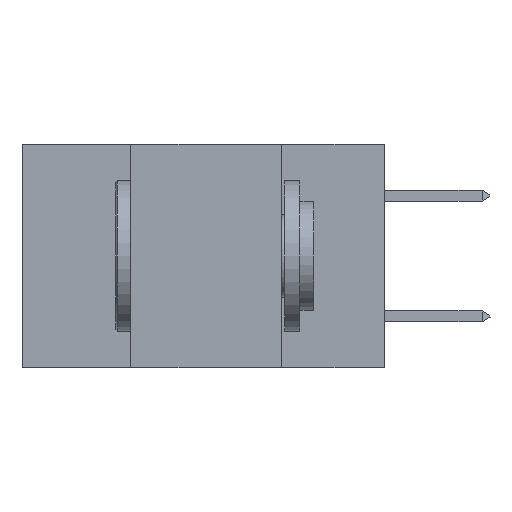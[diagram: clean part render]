
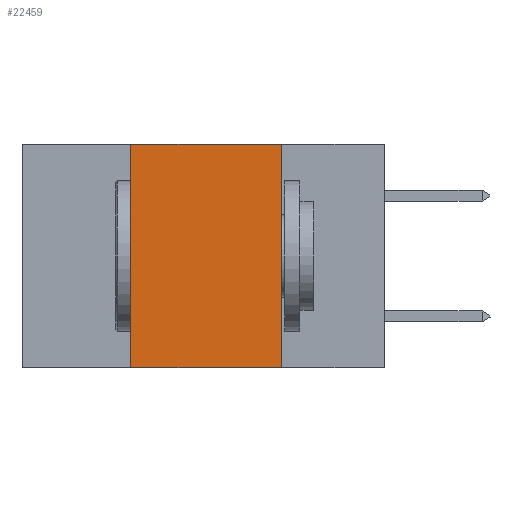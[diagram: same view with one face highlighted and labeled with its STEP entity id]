
A CAD part, left-side view. The second image highlights one B-rep face of the part: STEP entity #22459.
In plain terms, the highlighted planar face has unit normal (-1, 0, 0).
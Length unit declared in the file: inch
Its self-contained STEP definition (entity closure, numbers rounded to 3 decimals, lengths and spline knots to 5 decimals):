
#873 = LINE ( 'NONE', #25288, #9762 ) ;
#1353 = EDGE_CURVE ( 'NONE', #3779, #5149, #873, .T. ) ;
#2006 = CARTESIAN_POINT ( 'NONE',  ( 0., 0.6, 0. ) ) ;
#2845 = VERTEX_POINT ( 'NONE', #12413 ) ;
#3779 = VERTEX_POINT ( 'NONE', #20628 ) ;
#4001 = EDGE_CURVE ( 'NONE', #22722, #3779, #24430, .T. ) ;
#5149 = VERTEX_POINT ( 'NONE', #20703 ) ;
#5752 = VECTOR ( 'NONE', #41455, 39.37008 ) ;
#6653 = DIRECTION ( 'NONE',  ( 0., 0., 1. ) ) ;
#9762 = VECTOR ( 'NONE', #21986, 39.37008 ) ;
#11736 = CARTESIAN_POINT ( 'NONE',  ( 0., 0.42, 0. ) ) ;
#12413 = CARTESIAN_POINT ( 'NONE',  ( 0., 0.42, -0.37 ) ) ;
#13778 = VECTOR ( 'NONE', #6653, 39.37008 ) ;
#14039 = PLANE ( 'NONE',  #39167 ) ;
#15725 = ORIENTED_EDGE ( 'NONE', *, *, #20161, .T. ) ;
#15850 = LINE ( 'NONE', #26395, #13778 ) ;
#18760 = ORIENTED_EDGE ( 'NONE', *, *, #4001, .F. ) ;
#20161 = EDGE_CURVE ( 'NONE', #2845, #5149, #31944, .T. ) ;
#20608 = DIRECTION ( 'NONE',  ( 0., 0., -1. ) ) ;
#20628 = CARTESIAN_POINT ( 'NONE',  ( 0., 0.17, 0. ) ) ;
#20703 = CARTESIAN_POINT ( 'NONE',  ( 0., 0.17, -0.37 ) ) ;
#21986 = DIRECTION ( 'NONE',  ( 0., 0., -1. ) ) ;
#22459 = ADVANCED_FACE ( 'NONE', ( #36259 ), #14039, .F. ) ;
#22722 = VERTEX_POINT ( 'NONE', #11736 ) ;
#23468 = EDGE_CURVE ( 'NONE', #2845, #22722, #15850, .T. ) ;
#23849 = ORIENTED_EDGE ( 'NONE', *, *, #1353, .F. ) ;
#24430 = LINE ( 'NONE', #2006, #41568 ) ;
#25088 = DIRECTION ( 'NONE',  ( 0., -1., 0. ) ) ;
#25288 = CARTESIAN_POINT ( 'NONE',  ( 0., 0.17, 0. ) ) ;
#26395 = CARTESIAN_POINT ( 'NONE',  ( 0., 0.42, 0. ) ) ;
#30049 = ORIENTED_EDGE ( 'NONE', *, *, #23468, .F. ) ;
#31944 = LINE ( 'NONE', #38211, #5752 ) ;
#36259 = FACE_OUTER_BOUND ( 'NONE', #40569, .T. ) ;
#36783 = CARTESIAN_POINT ( 'NONE',  ( 0., 0.6, 0. ) ) ;
#38211 = CARTESIAN_POINT ( 'NONE',  ( 0., 0.6, -0.37 ) ) ;
#39167 = AXIS2_PLACEMENT_3D ( 'NONE', #36783, #40004, #20608 ) ;
#40004 = DIRECTION ( 'NONE',  ( 1., 0., 0. ) ) ;
#40569 = EDGE_LOOP ( 'NONE', ( #23849, #18760, #30049, #15725 ) ) ;
#41455 = DIRECTION ( 'NONE',  ( 0., -1., 0. ) ) ;
#41568 = VECTOR ( 'NONE', #25088, 39.37008 ) ;
